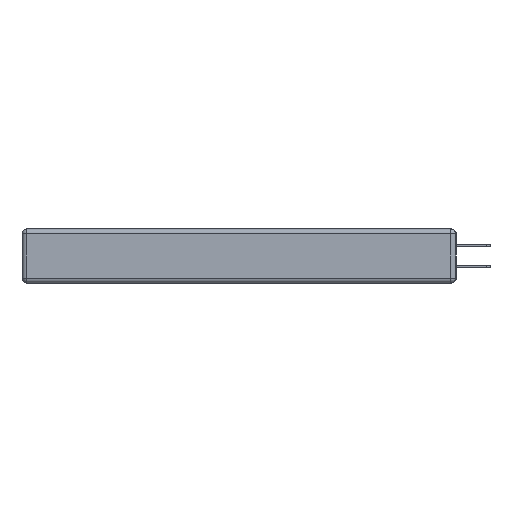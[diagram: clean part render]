
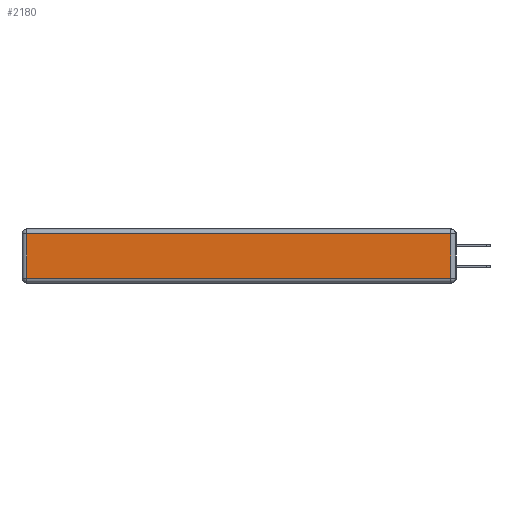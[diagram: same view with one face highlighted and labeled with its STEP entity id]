
A CAD part, left-side view. The second image highlights one B-rep face of the part: STEP entity #2180.
In plain terms, the highlighted planar face has unit normal (-1, 0, 0).
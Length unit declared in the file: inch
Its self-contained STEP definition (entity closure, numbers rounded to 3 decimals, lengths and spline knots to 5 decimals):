
#891 = DIRECTION ( 'NONE',  ( -1., 0., 0. ) ) ;
#919 = EDGE_CURVE ( 'NONE', #4374, #9758, #4349, .T. ) ;
#1084 = VECTOR ( 'NONE', #7393, 39.37008 ) ;
#1268 = CARTESIAN_POINT ( 'NONE',  ( 0., 0.03, -0.03 ) ) ;
#2180 = ADVANCED_FACE ( 'NONE', ( #11005 ), #6123, .T. ) ;
#2581 = EDGE_CURVE ( 'NONE', #9758, #8858, #16583, .T. ) ;
#3546 = VECTOR ( 'NONE', #20981, 39.37008 ) ;
#4349 = LINE ( 'NONE', #21126, #3546 ) ;
#4374 = VERTEX_POINT ( 'NONE', #17196 ) ;
#4456 = EDGE_LOOP ( 'NONE', ( #16907, #14880, #16407, #18865 ) ) ;
#6123 = PLANE ( 'NONE',  #15939 ) ;
#6756 = EDGE_CURVE ( 'NONE', #22001, #4374, #16441, .T. ) ;
#7393 = DIRECTION ( 'NONE',  ( 0., 1., 0. ) ) ;
#7863 = CARTESIAN_POINT ( 'NONE',  ( 0., 0., -0.343 ) ) ;
#8416 = VECTOR ( 'NONE', #20359, 39.37008 ) ;
#8858 = VERTEX_POINT ( 'NONE', #13172 ) ;
#9495 = DIRECTION ( 'NONE',  ( 0., 0., 1. ) ) ;
#9542 = CARTESIAN_POINT ( 'NONE',  ( 0., 2.72, -0.343 ) ) ;
#9758 = VERTEX_POINT ( 'NONE', #1268 ) ;
#10742 = VECTOR ( 'NONE', #18307, 39.37008 ) ;
#11005 = FACE_OUTER_BOUND ( 'NONE', #4456, .T. ) ;
#12828 = CARTESIAN_POINT ( 'NONE',  ( 0., 2.72, -0.313 ) ) ;
#13172 = CARTESIAN_POINT ( 'NONE',  ( 0., 2.72, -0.03 ) ) ;
#14880 = ORIENTED_EDGE ( 'NONE', *, *, #919, .T. ) ;
#15939 = AXIS2_PLACEMENT_3D ( 'NONE', #7863, #891, #9495 ) ;
#16407 = ORIENTED_EDGE ( 'NONE', *, *, #2581, .T. ) ;
#16441 = LINE ( 'NONE', #17122, #8416 ) ;
#16583 = LINE ( 'NONE', #17615, #1084 ) ;
#16907 = ORIENTED_EDGE ( 'NONE', *, *, #6756, .T. ) ;
#17122 = CARTESIAN_POINT ( 'NONE',  ( 0., 0., -0.313 ) ) ;
#17196 = CARTESIAN_POINT ( 'NONE',  ( 0., 0.03, -0.313 ) ) ;
#17615 = CARTESIAN_POINT ( 'NONE',  ( 0., 2.75, -0.03 ) ) ;
#17665 = LINE ( 'NONE', #9542, #10742 ) ;
#18307 = DIRECTION ( 'NONE',  ( 0., 0., -1. ) ) ;
#18865 = ORIENTED_EDGE ( 'NONE', *, *, #19456, .T. ) ;
#19456 = EDGE_CURVE ( 'NONE', #8858, #22001, #17665, .T. ) ;
#20359 = DIRECTION ( 'NONE',  ( 0., -1., 0. ) ) ;
#20981 = DIRECTION ( 'NONE',  ( 0., 0., 1. ) ) ;
#21126 = CARTESIAN_POINT ( 'NONE',  ( 0., 0.03, -0.343 ) ) ;
#22001 = VERTEX_POINT ( 'NONE', #12828 ) ;
